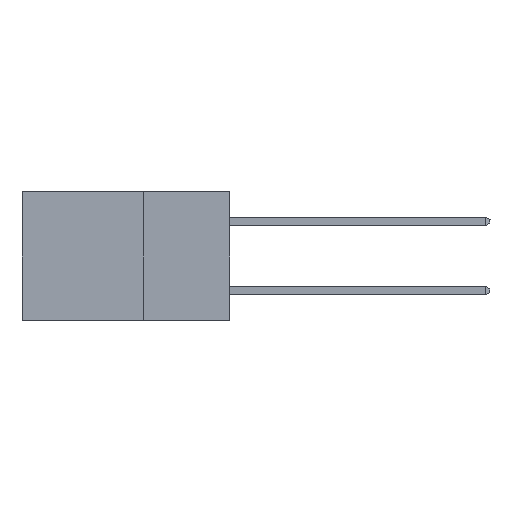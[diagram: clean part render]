
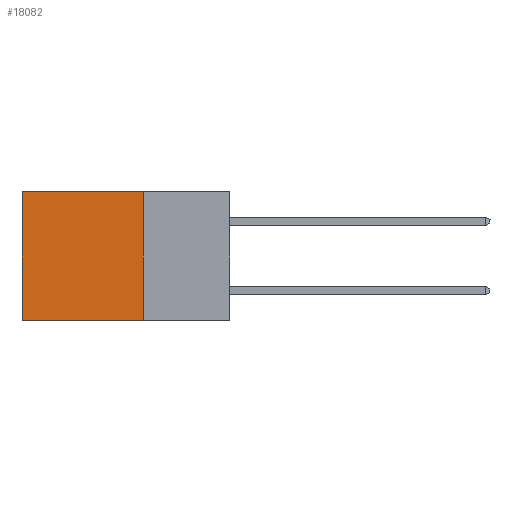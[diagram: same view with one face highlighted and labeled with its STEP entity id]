
A CAD part, left-side view. The second image highlights one B-rep face of the part: STEP entity #18082.
In plain terms, the highlighted planar face has unit normal (-1, 0, 0).
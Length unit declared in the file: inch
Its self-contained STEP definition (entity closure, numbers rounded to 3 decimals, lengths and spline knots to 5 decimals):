
#291 = ORIENTED_EDGE ( 'NONE', *, *, #13529, .F. ) ;
#1322 = EDGE_LOOP ( 'NONE', ( #3431, #2570, #291, #3714 ) ) ;
#2381 = DIRECTION ( 'NONE',  ( 1., 0., 0. ) ) ;
#2570 = ORIENTED_EDGE ( 'NONE', *, *, #3268, .F. ) ;
#2822 = VECTOR ( 'NONE', #7411, 39.37008 ) ;
#3268 = EDGE_CURVE ( 'NONE', #11490, #6987, #7527, .T. ) ;
#3431 = ORIENTED_EDGE ( 'NONE', *, *, #17528, .T. ) ;
#3714 = ORIENTED_EDGE ( 'NONE', *, *, #10356, .T. ) ;
#4325 = FACE_OUTER_BOUND ( 'NONE', #1322, .T. ) ;
#4358 = CARTESIAN_POINT ( 'NONE',  ( 0.2615, 0.6, -0.37 ) ) ;
#6075 = VECTOR ( 'NONE', #13527, 39.37008 ) ;
#6309 = CARTESIAN_POINT ( 'NONE',  ( 0.2615, 0.25, 0. ) ) ;
#6987 = VERTEX_POINT ( 'NONE', #9728 ) ;
#7411 = DIRECTION ( 'NONE',  ( 0., 0., -1. ) ) ;
#7527 = LINE ( 'NONE', #11444, #6075 ) ;
#9728 = CARTESIAN_POINT ( 'NONE',  ( 0.2615, 0.6, -0.37 ) ) ;
#10356 = EDGE_CURVE ( 'NONE', #23305, #15466, #13583, .T. ) ;
#10469 = CARTESIAN_POINT ( 'NONE',  ( 0.2615, 0.25, -0.37 ) ) ;
#11444 = CARTESIAN_POINT ( 'NONE',  ( 0.2615, 0.25, -0.37 ) ) ;
#11490 = VERTEX_POINT ( 'NONE', #18547 ) ;
#11644 = DIRECTION ( 'NONE',  ( 0., 1., 0. ) ) ;
#12687 = VECTOR ( 'NONE', #20235, 39.37008 ) ;
#13527 = DIRECTION ( 'NONE',  ( 0., 1., 0. ) ) ;
#13529 = EDGE_CURVE ( 'NONE', #23305, #11490, #25220, .T. ) ;
#13583 = LINE ( 'NONE', #21630, #23096 ) ;
#15466 = VERTEX_POINT ( 'NONE', #16356 ) ;
#16356 = CARTESIAN_POINT ( 'NONE',  ( 0.2615, 0.6, 0. ) ) ;
#17446 = CARTESIAN_POINT ( 'NONE',  ( 0.2615, 0.25, -0.37 ) ) ;
#17528 = EDGE_CURVE ( 'NONE', #15466, #6987, #22176, .T. ) ;
#17676 = AXIS2_PLACEMENT_3D ( 'NONE', #10469, #2381, #24216 ) ;
#18082 = ADVANCED_FACE ( 'NONE', ( #4325 ), #20194, .F. ) ;
#18547 = CARTESIAN_POINT ( 'NONE',  ( 0.2615, 0.25, -0.37 ) ) ;
#20194 = PLANE ( 'NONE',  #17676 ) ;
#20235 = DIRECTION ( 'NONE',  ( 0., 0., -1. ) ) ;
#21630 = CARTESIAN_POINT ( 'NONE',  ( 0.2615, 0.25, 0. ) ) ;
#22176 = LINE ( 'NONE', #4358, #12687 ) ;
#23096 = VECTOR ( 'NONE', #11644, 39.37008 ) ;
#23305 = VERTEX_POINT ( 'NONE', #6309 ) ;
#24216 = DIRECTION ( 'NONE',  ( 0., 0., -1. ) ) ;
#25220 = LINE ( 'NONE', #17446, #2822 ) ;
